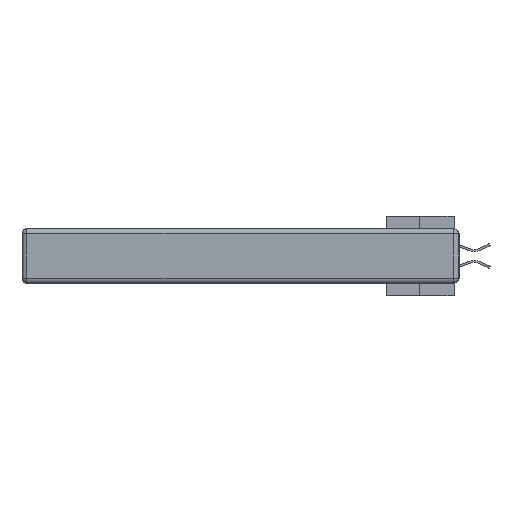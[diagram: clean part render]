
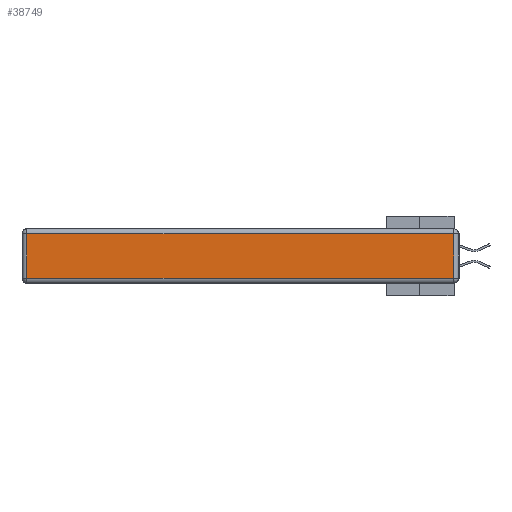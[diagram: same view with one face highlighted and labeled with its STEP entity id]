
A CAD part, left-side view. The second image highlights one B-rep face of the part: STEP entity #38749.
In plain terms, the highlighted planar face has unit normal (-1, 0, 0).
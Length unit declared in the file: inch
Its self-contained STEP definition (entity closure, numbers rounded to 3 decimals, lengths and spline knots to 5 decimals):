
#2205 = EDGE_CURVE ( 'NONE', #47506, #41967, #30987, .T. ) ;
#3977 = CARTESIAN_POINT ( 'NONE',  ( 0., 0., -0.343 ) ) ;
#4133 = VERTEX_POINT ( 'NONE', #16790 ) ;
#5041 = DIRECTION ( 'NONE',  ( 0., 0., 1. ) ) ;
#5183 = ORIENTED_EDGE ( 'NONE', *, *, #16582, .T. ) ;
#10234 = CARTESIAN_POINT ( 'NONE',  ( 0., 0.03, -0.03 ) ) ;
#10502 = DIRECTION ( 'NONE',  ( 0., 1., 0. ) ) ;
#13472 = VERTEX_POINT ( 'NONE', #45362 ) ;
#13845 = VECTOR ( 'NONE', #24511, 39.37008 ) ;
#16285 = EDGE_CURVE ( 'NONE', #4133, #47506, #46664, .T. ) ;
#16582 = EDGE_CURVE ( 'NONE', #13472, #4133, #19595, .T. ) ;
#16790 = CARTESIAN_POINT ( 'NONE',  ( 0., 2.72, -0.313 ) ) ;
#17666 = LINE ( 'NONE', #29117, #46202 ) ;
#19257 = PLANE ( 'NONE',  #37598 ) ;
#19595 = LINE ( 'NONE', #33773, #30187 ) ;
#20351 = VECTOR ( 'NONE', #5041, 39.37008 ) ;
#20870 = FACE_OUTER_BOUND ( 'NONE', #28522, .T. ) ;
#23219 = DIRECTION ( 'NONE',  ( 0., 0., 1. ) ) ;
#24511 = DIRECTION ( 'NONE',  ( 0., -1., 0. ) ) ;
#28148 = CARTESIAN_POINT ( 'NONE',  ( 0., 0.03, -0.313 ) ) ;
#28522 = EDGE_LOOP ( 'NONE', ( #35279, #43703, #31201, #5183 ) ) ;
#29117 = CARTESIAN_POINT ( 'NONE',  ( 0., 2.75, -0.03 ) ) ;
#30139 = DIRECTION ( 'NONE',  ( 0., 0., -1. ) ) ;
#30187 = VECTOR ( 'NONE', #30139, 39.37008 ) ;
#30987 = LINE ( 'NONE', #38810, #20351 ) ;
#31201 = ORIENTED_EDGE ( 'NONE', *, *, #38057, .T. ) ;
#33773 = CARTESIAN_POINT ( 'NONE',  ( 0., 2.72, -0.343 ) ) ;
#35279 = ORIENTED_EDGE ( 'NONE', *, *, #16285, .T. ) ;
#37598 = AXIS2_PLACEMENT_3D ( 'NONE', #3977, #45701, #23219 ) ;
#38057 = EDGE_CURVE ( 'NONE', #41967, #13472, #17666, .T. ) ;
#38749 = ADVANCED_FACE ( 'NONE', ( #20870 ), #19257, .T. ) ;
#38810 = CARTESIAN_POINT ( 'NONE',  ( 0., 0.03, -0.343 ) ) ;
#39963 = CARTESIAN_POINT ( 'NONE',  ( 0., 0., -0.313 ) ) ;
#41967 = VERTEX_POINT ( 'NONE', #10234 ) ;
#43703 = ORIENTED_EDGE ( 'NONE', *, *, #2205, .T. ) ;
#45362 = CARTESIAN_POINT ( 'NONE',  ( 0., 2.72, -0.03 ) ) ;
#45701 = DIRECTION ( 'NONE',  ( -1., 0., 0. ) ) ;
#46202 = VECTOR ( 'NONE', #10502, 39.37008 ) ;
#46664 = LINE ( 'NONE', #39963, #13845 ) ;
#47506 = VERTEX_POINT ( 'NONE', #28148 ) ;
